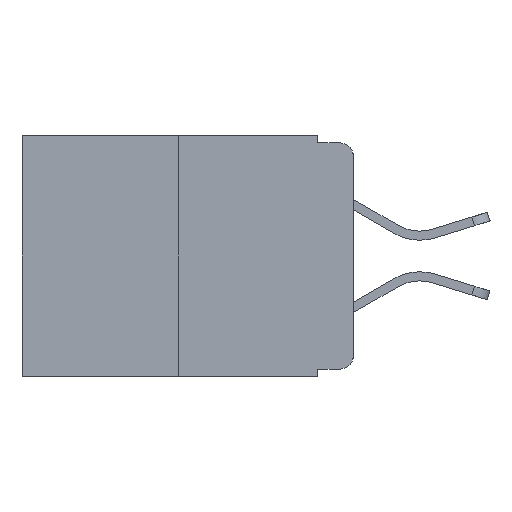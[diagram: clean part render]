
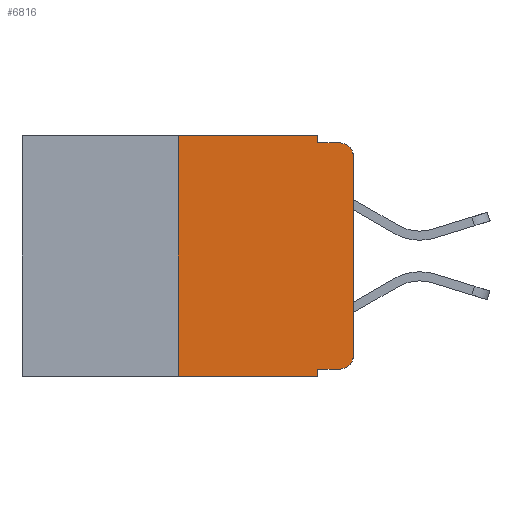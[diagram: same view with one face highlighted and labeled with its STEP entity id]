
A CAD part, left-side view. The second image highlights one B-rep face of the part: STEP entity #6816.
In plain terms, the highlighted planar face has unit normal (-1, 0, 0).
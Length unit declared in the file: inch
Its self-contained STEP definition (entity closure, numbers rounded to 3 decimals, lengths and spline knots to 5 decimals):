
#336 = VERTEX_POINT ( 'NONE', #7704 ) ;
#344 = VECTOR ( 'NONE', #931, 39.37008 ) ;
#353 = AXIS2_PLACEMENT_3D ( 'NONE', #12138, #2159, #2114 ) ;
#457 = VERTEX_POINT ( 'NONE', #13073 ) ;
#558 = CARTESIAN_POINT ( 'NONE',  ( 0., 0.25, 0. ) ) ;
#635 = VERTEX_POINT ( 'NONE', #2987 ) ;
#723 = CARTESIAN_POINT ( 'NONE',  ( 0., 0.02, -0.03 ) ) ;
#832 = AXIS2_PLACEMENT_3D ( 'NONE', #19618, #16662, #7402 ) ;
#864 = LINE ( 'NONE', #5651, #344 ) ;
#931 = DIRECTION ( 'NONE',  ( 0., 0., -1. ) ) ;
#1638 = LINE ( 'NONE', #19654, #5376 ) ;
#1812 = LINE ( 'NONE', #15242, #17866 ) ;
#2094 = CIRCLE ( 'NONE', #20201, 0.02 ) ;
#2114 = DIRECTION ( 'NONE',  ( 0., 0., -1. ) ) ;
#2153 = ORIENTED_EDGE ( 'NONE', *, *, #16693, .F. ) ;
#2159 = DIRECTION ( 'NONE',  ( -1., 0., 0. ) ) ;
#2356 = CARTESIAN_POINT ( 'NONE',  ( 0., 0.25, 0. ) ) ;
#2366 = DIRECTION ( 'NONE',  ( 0., 0., -1. ) ) ;
#2394 = CARTESIAN_POINT ( 'NONE',  ( 0., 0.051, -0.01 ) ) ;
#2501 = EDGE_CURVE ( 'NONE', #19415, #11635, #9889, .T. ) ;
#2987 = CARTESIAN_POINT ( 'NONE',  ( 0., 0., -0.03 ) ) ;
#3397 = DIRECTION ( 'NONE',  ( 0., -1., 0. ) ) ;
#3418 = ORIENTED_EDGE ( 'NONE', *, *, #15216, .F. ) ;
#3444 = VERTEX_POINT ( 'NONE', #15920 ) ;
#3935 = EDGE_CURVE ( 'NONE', #4454, #3444, #864, .T. ) ;
#4275 = DIRECTION ( 'NONE',  ( 0., -1., 0. ) ) ;
#4294 = DIRECTION ( 'NONE',  ( 0., 0., 1. ) ) ;
#4415 = CARTESIAN_POINT ( 'NONE',  ( 0., 0.051, -0.333 ) ) ;
#4454 = VERTEX_POINT ( 'NONE', #4415 ) ;
#5376 = VECTOR ( 'NONE', #4294, 39.37008 ) ;
#5523 = VERTEX_POINT ( 'NONE', #2394 ) ;
#5651 = CARTESIAN_POINT ( 'NONE',  ( 0., 0.051, 0. ) ) ;
#5677 = EDGE_CURVE ( 'NONE', #336, #3444, #1812, .T. ) ;
#5828 = CARTESIAN_POINT ( 'NONE',  ( 0., 0.051, 0. ) ) ;
#6746 = FACE_OUTER_BOUND ( 'NONE', #14079, .T. ) ;
#6780 = CARTESIAN_POINT ( 'NONE',  ( 0., 0.051, -0.333 ) ) ;
#6816 = ADVANCED_FACE ( 'NONE', ( #6746 ), #13581, .F. ) ;
#6881 = ORIENTED_EDGE ( 'NONE', *, *, #16224, .F. ) ;
#7402 = DIRECTION ( 'NONE',  ( 0., 0., -1. ) ) ;
#7437 = EDGE_CURVE ( 'NONE', #4454, #19415, #7948, .T. ) ;
#7443 = VECTOR ( 'NONE', #9951, 39.37008 ) ;
#7490 = LINE ( 'NONE', #5828, #15717 ) ;
#7704 = CARTESIAN_POINT ( 'NONE',  ( 0., 0.25, -0.343 ) ) ;
#7948 = LINE ( 'NONE', #6780, #7443 ) ;
#8151 = CARTESIAN_POINT ( 'NONE',  ( 0., 0.051, 0. ) ) ;
#8365 = ORIENTED_EDGE ( 'NONE', *, *, #14274, .T. ) ;
#9105 = DIRECTION ( 'NONE',  ( 0., -1., 0. ) ) ;
#9889 = CIRCLE ( 'NONE', #353, 0.02 ) ;
#9951 = DIRECTION ( 'NONE',  ( 0., -1., 0. ) ) ;
#10096 = ORIENTED_EDGE ( 'NONE', *, *, #14783, .T. ) ;
#10206 = VERTEX_POINT ( 'NONE', #8151 ) ;
#10372 = CARTESIAN_POINT ( 'NONE',  ( 0., 0.02, -0.333 ) ) ;
#10444 = CARTESIAN_POINT ( 'NONE',  ( 0., 0., -0.313 ) ) ;
#10534 = CARTESIAN_POINT ( 'NONE',  ( 0., 0.473, 0. ) ) ;
#10677 = VECTOR ( 'NONE', #11644, 39.37008 ) ;
#11435 = ORIENTED_EDGE ( 'NONE', *, *, #2501, .T. ) ;
#11635 = VERTEX_POINT ( 'NONE', #10444 ) ;
#11644 = DIRECTION ( 'NONE',  ( 0., 0., 1. ) ) ;
#11795 = DIRECTION ( 'NONE',  ( -1., 0., 0. ) ) ;
#12138 = CARTESIAN_POINT ( 'NONE',  ( 0., 0.02, -0.313 ) ) ;
#12236 = ORIENTED_EDGE ( 'NONE', *, *, #17993, .F. ) ;
#13073 = CARTESIAN_POINT ( 'NONE',  ( 0., 0.02, -0.01 ) ) ;
#13581 = PLANE ( 'NONE',  #832 ) ;
#13740 = LINE ( 'NONE', #10534, #17311 ) ;
#13833 = ORIENTED_EDGE ( 'NONE', *, *, #7437, .T. ) ;
#14078 = VECTOR ( 'NONE', #3397, 39.37008 ) ;
#14079 = EDGE_LOOP ( 'NONE', ( #8365, #10096, #3418, #6881, #12236, #2153, #18396, #15824, #13833, #11435 ) ) ;
#14274 = EDGE_CURVE ( 'NONE', #11635, #635, #1638, .T. ) ;
#14783 = EDGE_CURVE ( 'NONE', #635, #457, #2094, .T. ) ;
#15216 = EDGE_CURVE ( 'NONE', #5523, #457, #18123, .T. ) ;
#15242 = CARTESIAN_POINT ( 'NONE',  ( 0., 0.473, -0.343 ) ) ;
#15717 = VECTOR ( 'NONE', #16671, 39.37008 ) ;
#15824 = ORIENTED_EDGE ( 'NONE', *, *, #3935, .F. ) ;
#15920 = CARTESIAN_POINT ( 'NONE',  ( 0., 0.051, -0.343 ) ) ;
#16224 = EDGE_CURVE ( 'NONE', #10206, #5523, #7490, .T. ) ;
#16662 = DIRECTION ( 'NONE',  ( 1., 0., 0. ) ) ;
#16671 = DIRECTION ( 'NONE',  ( 0., 0., -1. ) ) ;
#16693 = EDGE_CURVE ( 'NONE', #336, #19377, #18757, .T. ) ;
#17311 = VECTOR ( 'NONE', #4275, 39.37008 ) ;
#17866 = VECTOR ( 'NONE', #9105, 39.37008 ) ;
#17993 = EDGE_CURVE ( 'NONE', #19377, #10206, #13740, .T. ) ;
#18123 = LINE ( 'NONE', #18818, #14078 ) ;
#18396 = ORIENTED_EDGE ( 'NONE', *, *, #5677, .T. ) ;
#18757 = LINE ( 'NONE', #558, #10677 ) ;
#18818 = CARTESIAN_POINT ( 'NONE',  ( 0., 0.051, -0.01 ) ) ;
#19377 = VERTEX_POINT ( 'NONE', #2356 ) ;
#19415 = VERTEX_POINT ( 'NONE', #10372 ) ;
#19618 = CARTESIAN_POINT ( 'NONE',  ( 0., 0.473, 0. ) ) ;
#19654 = CARTESIAN_POINT ( 'NONE',  ( 0., 0., 0. ) ) ;
#20201 = AXIS2_PLACEMENT_3D ( 'NONE', #723, #11795, #2366 ) ;
